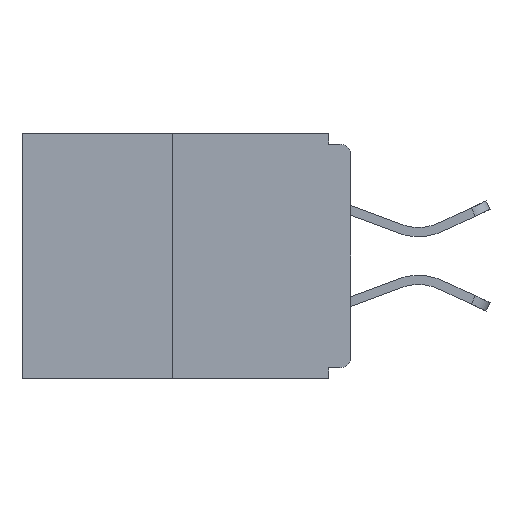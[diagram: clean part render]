
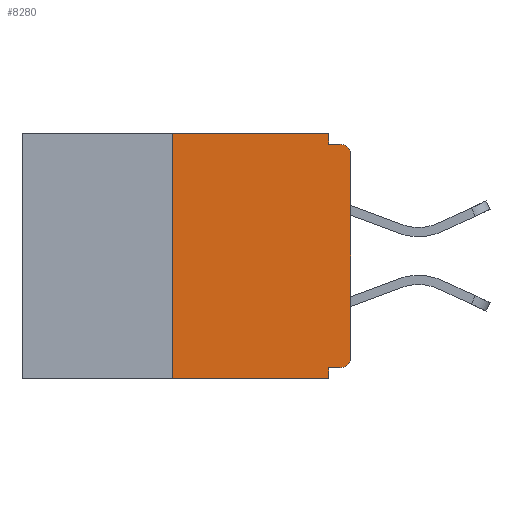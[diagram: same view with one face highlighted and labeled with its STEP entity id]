
A CAD part, left-side view. The second image highlights one B-rep face of the part: STEP entity #8280.
In plain terms, the highlighted planar face has unit normal (-1, 0, 0).
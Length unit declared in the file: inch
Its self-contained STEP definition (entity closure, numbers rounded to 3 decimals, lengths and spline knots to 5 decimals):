
#9 = EDGE_LOOP ( 'NONE', ( #11543, #6482, #7509, #4244, #10750, #7469, #377, #11772, #1000, #10721 ) ) ;
#377 = ORIENTED_EDGE ( 'NONE', *, *, #4257, .T. ) ;
#393 = FACE_OUTER_BOUND ( 'NONE', #9, .T. ) ;
#716 = VERTEX_POINT ( 'NONE', #4046 ) ;
#769 = VECTOR ( 'NONE', #13009, 39.37008 ) ;
#959 = VERTEX_POINT ( 'NONE', #8981 ) ;
#1000 = ORIENTED_EDGE ( 'NONE', *, *, #1274, .F. ) ;
#1040 = DIRECTION ( 'NONE',  ( 0., 1., 0. ) ) ;
#1081 = DIRECTION ( 'NONE',  ( -1., 0., 0. ) ) ;
#1195 = DIRECTION ( 'NONE',  ( -1., 0., 0. ) ) ;
#1274 = EDGE_CURVE ( 'NONE', #8501, #959, #8161, .T. ) ;
#1825 = CARTESIAN_POINT ( 'NONE',  ( 0., 0.46, 0. ) ) ;
#1831 = VECTOR ( 'NONE', #9952, 39.37008 ) ;
#2010 = LINE ( 'NONE', #2644, #1831 ) ;
#2164 = CARTESIAN_POINT ( 'NONE',  ( 0., 0., -0.328 ) ) ;
#2544 = VECTOR ( 'NONE', #6249, 39.37008 ) ;
#2581 = CARTESIAN_POINT ( 'NONE',  ( 0., 0., -0.03 ) ) ;
#2644 = CARTESIAN_POINT ( 'NONE',  ( 0., 0.031, 0. ) ) ;
#2712 = DIRECTION ( 'NONE',  ( 0., -1., 0. ) ) ;
#2852 = VECTOR ( 'NONE', #6536, 39.37008 ) ;
#3035 = VERTEX_POINT ( 'NONE', #2581 ) ;
#3160 = EDGE_CURVE ( 'NONE', #10809, #3625, #11036, .T. ) ;
#3278 = AXIS2_PLACEMENT_3D ( 'NONE', #11488, #1081, #11443 ) ;
#3625 = VERTEX_POINT ( 'NONE', #10145 ) ;
#3684 = CARTESIAN_POINT ( 'NONE',  ( 0., 0., -0.015 ) ) ;
#3698 = PLANE ( 'NONE',  #11601 ) ;
#3903 = EDGE_CURVE ( 'NONE', #4562, #8880, #9212, .T. ) ;
#4046 = CARTESIAN_POINT ( 'NONE',  ( 0., 0.031, 0. ) ) ;
#4092 = EDGE_CURVE ( 'NONE', #12812, #4562, #7756, .T. ) ;
#4244 = ORIENTED_EDGE ( 'NONE', *, *, #3903, .F. ) ;
#4257 = EDGE_CURVE ( 'NONE', #5837, #3035, #6615, .T. ) ;
#4562 = VERTEX_POINT ( 'NONE', #6519 ) ;
#4807 = LINE ( 'NONE', #8918, #10513 ) ;
#4989 = CARTESIAN_POINT ( 'NONE',  ( 0., 0.25, -0.343 ) ) ;
#5504 = CARTESIAN_POINT ( 'NONE',  ( 0., 0., 0. ) ) ;
#5785 = DIRECTION ( 'NONE',  ( 0., -1., 0. ) ) ;
#5837 = VERTEX_POINT ( 'NONE', #10478 ) ;
#6249 = DIRECTION ( 'NONE',  ( 0., 0., -1. ) ) ;
#6482 = ORIENTED_EDGE ( 'NONE', *, *, #3160, .F. ) ;
#6519 = CARTESIAN_POINT ( 'NONE',  ( 0., 0.031, -0.328 ) ) ;
#6536 = DIRECTION ( 'NONE',  ( 0., 0., 1. ) ) ;
#6615 = LINE ( 'NONE', #5504, #2852 ) ;
#6665 = VECTOR ( 'NONE', #10092, 39.37008 ) ;
#6828 = CARTESIAN_POINT ( 'NONE',  ( 0., 0.46, 0. ) ) ;
#7257 = EDGE_CURVE ( 'NONE', #10809, #8880, #4807, .T. ) ;
#7469 = ORIENTED_EDGE ( 'NONE', *, *, #9921, .T. ) ;
#7509 = ORIENTED_EDGE ( 'NONE', *, *, #7257, .T. ) ;
#7686 = CARTESIAN_POINT ( 'NONE',  ( 0., 0.031, -0.015 ) ) ;
#7718 = CARTESIAN_POINT ( 'NONE',  ( 0., 0.015, -0.328 ) ) ;
#7756 = LINE ( 'NONE', #2164, #9720 ) ;
#7757 = AXIS2_PLACEMENT_3D ( 'NONE', #10715, #1195, #10585 ) ;
#7945 = CIRCLE ( 'NONE', #7757, 0.015 ) ;
#8161 = LINE ( 'NONE', #3684, #12679 ) ;
#8280 = ADVANCED_FACE ( 'NONE', ( #393 ), #3698, .F. ) ;
#8501 = VERTEX_POINT ( 'NONE', #7686 ) ;
#8880 = VERTEX_POINT ( 'NONE', #12527 ) ;
#8918 = CARTESIAN_POINT ( 'NONE',  ( 0., 0.46, -0.343 ) ) ;
#8981 = CARTESIAN_POINT ( 'NONE',  ( 0., 0.015, -0.015 ) ) ;
#9006 = CARTESIAN_POINT ( 'NONE',  ( 0., 0.25, 0. ) ) ;
#9212 = LINE ( 'NONE', #9344, #2544 ) ;
#9344 = CARTESIAN_POINT ( 'NONE',  ( 0., 0.031, -0.343 ) ) ;
#9720 = VECTOR ( 'NONE', #1040, 39.37008 ) ;
#9861 = DIRECTION ( 'NONE',  ( 0., 0., -1. ) ) ;
#9921 = EDGE_CURVE ( 'NONE', #12812, #5837, #10115, .T. ) ;
#9952 = DIRECTION ( 'NONE',  ( 0., 0., -1. ) ) ;
#10092 = DIRECTION ( 'NONE',  ( 0., -1., 0. ) ) ;
#10115 = CIRCLE ( 'NONE', #3278, 0.015 ) ;
#10145 = CARTESIAN_POINT ( 'NONE',  ( 0., 0.25, 0. ) ) ;
#10478 = CARTESIAN_POINT ( 'NONE',  ( 0., 0., -0.313 ) ) ;
#10513 = VECTOR ( 'NONE', #2712, 39.37008 ) ;
#10585 = DIRECTION ( 'NONE',  ( 0., 0., -1. ) ) ;
#10607 = EDGE_CURVE ( 'NONE', #3625, #716, #13133, .T. ) ;
#10715 = CARTESIAN_POINT ( 'NONE',  ( 0., 0.015, -0.03 ) ) ;
#10721 = ORIENTED_EDGE ( 'NONE', *, *, #12793, .F. ) ;
#10750 = ORIENTED_EDGE ( 'NONE', *, *, #4092, .F. ) ;
#10809 = VERTEX_POINT ( 'NONE', #4989 ) ;
#10928 = DIRECTION ( 'NONE',  ( 1., 0., 0. ) ) ;
#11036 = LINE ( 'NONE', #9006, #769 ) ;
#11443 = DIRECTION ( 'NONE',  ( 0., 0., -1. ) ) ;
#11488 = CARTESIAN_POINT ( 'NONE',  ( 0., 0.015, -0.313 ) ) ;
#11543 = ORIENTED_EDGE ( 'NONE', *, *, #10607, .F. ) ;
#11601 = AXIS2_PLACEMENT_3D ( 'NONE', #6828, #10928, #9861 ) ;
#11772 = ORIENTED_EDGE ( 'NONE', *, *, #12078, .T. ) ;
#12078 = EDGE_CURVE ( 'NONE', #3035, #959, #7945, .T. ) ;
#12527 = CARTESIAN_POINT ( 'NONE',  ( 0., 0.031, -0.343 ) ) ;
#12679 = VECTOR ( 'NONE', #5785, 39.37008 ) ;
#12793 = EDGE_CURVE ( 'NONE', #716, #8501, #2010, .T. ) ;
#12812 = VERTEX_POINT ( 'NONE', #7718 ) ;
#13009 = DIRECTION ( 'NONE',  ( 0., 0., 1. ) ) ;
#13133 = LINE ( 'NONE', #1825, #6665 ) ;
